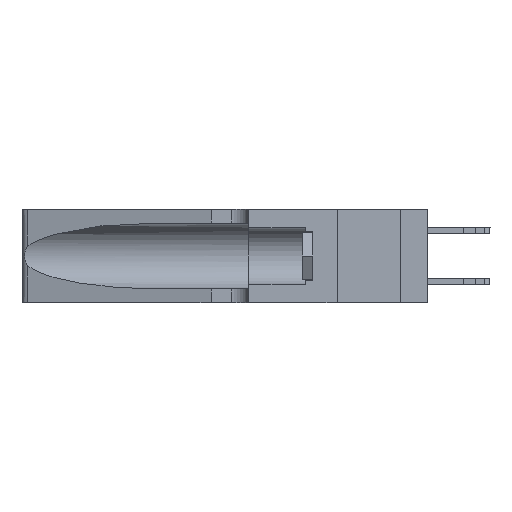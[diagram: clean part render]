
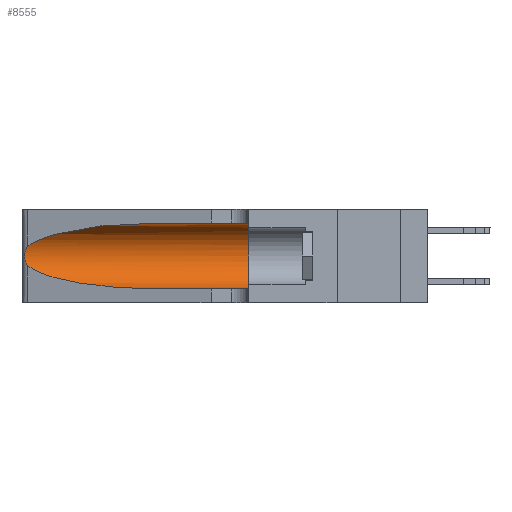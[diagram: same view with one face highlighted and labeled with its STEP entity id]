
A CAD part, left-side view. The second image highlights one B-rep face of the part: STEP entity #8555.
In plain terms, the highlighted cylindrical face has radius 3.308 mm (diameter 6.617 mm), a partial arc.
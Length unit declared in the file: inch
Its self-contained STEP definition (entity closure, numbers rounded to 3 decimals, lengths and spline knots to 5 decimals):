
#260 = CARTESIAN_POINT ( 'NONE',  ( 0.25639, 1.23186, 0.15144 ) ) ;
#756 = AXIS2_PLACEMENT_3D ( 'NONE', #12316, #9847, #24020 ) ;
#944 = VECTOR ( 'NONE', #30191, 39.37008 ) ;
#1982 = EDGE_CURVE ( 'NONE', #26042, #21639, #18127, .T. ) ;
#2422 = CARTESIAN_POINT ( 'NONE',  ( 0.25787, 1.23484, 0.2124 ) ) ;
#2727 = CARTESIAN_POINT ( 'NONE',  ( 0.25639, 1.23184, 0.21858 ) ) ;
#3432 = FACE_OUTER_BOUND ( 'NONE', #24597, .T. ) ;
#3894 = VERTEX_POINT ( 'NONE', #22502 ) ;
#4821 = CARTESIAN_POINT ( 'NONE',  ( 0.26075, 1.23896, 0.178 ) ) ;
#6118 = EDGE_CURVE ( 'NONE', #26042, #29046, #21059, .T. ) ;
#6675 = CARTESIAN_POINT ( 'NONE',  ( 0.2373, 1.15595, 0.28018 ) ) ;
#7386 = CARTESIAN_POINT ( 'NONE',  ( 0.25555, 1.22994, 0.2215 ) ) ;
#7749 = DIRECTION ( 'NONE',  ( 0., 0., -1. ) ) ;
#8228 = CARTESIAN_POINT ( 'NONE',  ( 0.1305, 0.72297, 0.31525 ) ) ;
#8555 = ADVANCED_FACE ( 'NONE', ( #3432 ), #15640, .F. ) ;
#9847 = DIRECTION ( 'NONE',  ( 0., 1., 0. ) ) ;
#10007 = VECTOR ( 'NONE', #13375, 39.37008 ) ;
#10968 = ORIENTED_EDGE ( 'NONE', *, *, #30305, .F. ) ;
#11940 = CARTESIAN_POINT ( 'NONE',  ( 0.26018, 1.23835, 0.19895 ) ) ;
#12041 = CARTESIAN_POINT ( 'NONE',  ( 0.26017, 1.23833, 0.17102 ) ) ;
#12077 = CARTESIAN_POINT ( 'NONE',  ( 0.25487, 1.22718, 0.22369 ) ) ;
#12197 = CARTESIAN_POINT ( 'NONE',  ( 0.2373, 1.15595, 0.08982 ) ) ;
#12316 = CARTESIAN_POINT ( 'NONE',  ( 0.1305, 0.35, 0.185 ) ) ;
#12512 = ORIENTED_EDGE ( 'NONE', *, *, #27457, .T. ) ;
#13101 = EDGE_CURVE ( 'NONE', #3894, #23990, #29773, .T. ) ;
#13375 = DIRECTION ( 'NONE',  ( 0., -1., 0. ) ) ;
#14307 = CARTESIAN_POINT ( 'NONE',  ( 0.25856, 1.23593, 0.16098 ) ) ;
#14887 = CARTESIAN_POINT ( 'NONE',  ( 0.1305, 1.61858, 0.185 ) ) ;
#14941 = ORIENTED_EDGE ( 'NONE', *, *, #13101, .T. ) ;
#15640 = CYLINDRICAL_SURFACE ( 'NONE', #25316, 0.13025 ) ;
#16698 = CARTESIAN_POINT ( 'NONE',  ( 0.25789, 1.23486, 0.15765 ) ) ;
#17646 = VERTEX_POINT ( 'NONE', #18879 ) ;
#18127 = LINE ( 'NONE', #25194, #10007 ) ;
#18879 = CARTESIAN_POINT ( 'NONE',  ( 0.1305, 0.35, 0.05475 ) ) ;
#19049 = B_SPLINE_CURVE_WITH_KNOTS ( 'NONE', 3,
 ( #28723, #7386, #2727, #2422, #19100, #11940, #19301, #4821, #12041, #14307, #16698, #260, #21687, #23845 ),
 .UNSPECIFIED., .F., .F.,
 ( 4, 2, 2, 2, 2, 2, 4 ),
 ( 0., 0.00027, 0.00053, 0.00107, 0.0016, 0.00187, 0.00214 ),
 .UNSPECIFIED. ) ;
#19100 = CARTESIAN_POINT ( 'NONE',  ( 0.25854, 1.2359, 0.20912 ) ) ;
#19301 = CARTESIAN_POINT ( 'NONE',  ( 0.26075, 1.23896, 0.19203 ) ) ;
#19317 = ORIENTED_EDGE ( 'NONE', *, *, #25510, .T. ) ;
#19349 = CARTESIAN_POINT ( 'NONE',  ( 0.18966, 0.96281, 0.05475 ) ) ;
#20085 = ORIENTED_EDGE ( 'NONE', *, *, #6118, .T. ) ;
#20572 = CARTESIAN_POINT ( 'NONE',  ( 0.1305, 1.61858, 0.05475 ) ) ;
#21059 =( BOUNDED_CURVE ( )  B_SPLINE_CURVE ( 3, ( #21366, #29432, #6675, #12077 ),
 .UNSPECIFIED., .F., .F. ) 
 B_SPLINE_CURVE_WITH_KNOTS ( ( 4, 4 ),
 ( 1.5708, 2.84003 ),
 .UNSPECIFIED. ) 
 CURVE ( )  GEOMETRIC_REPRESENTATION_ITEM ( )  RATIONAL_B_SPLINE_CURVE ( ( 1., 0.87, 0.87, 1. ) ) 
 REPRESENTATION_ITEM ( '' )  );
#21066 = CARTESIAN_POINT ( 'NONE',  ( 0.1305, 0.35, 0.31525 ) ) ;
#21366 = CARTESIAN_POINT ( 'NONE',  ( 0.1305, 0.72297, 0.31525 ) ) ;
#21639 = VERTEX_POINT ( 'NONE', #21066 ) ;
#21687 = CARTESIAN_POINT ( 'NONE',  ( 0.25555, 1.22993, 0.14849 ) ) ;
#22040 = DIRECTION ( 'NONE',  ( 0., -1., 0. ) ) ;
#22502 = CARTESIAN_POINT ( 'NONE',  ( 0.25487, 1.22718, 0.14631 ) ) ;
#22517 = CARTESIAN_POINT ( 'NONE',  ( 0.1305, 0.72297, 0.05475 ) ) ;
#23600 = ORIENTED_EDGE ( 'NONE', *, *, #1982, .F. ) ;
#23845 = CARTESIAN_POINT ( 'NONE',  ( 0.25487, 1.22718, 0.14631 ) ) ;
#23990 = VERTEX_POINT ( 'NONE', #22517 ) ;
#24020 = DIRECTION ( 'NONE',  ( 0., 0., 1. ) ) ;
#24597 = EDGE_LOOP ( 'NONE', ( #20085, #12512, #14941, #19317, #10968, #23600 ) ) ;
#25128 = CARTESIAN_POINT ( 'NONE',  ( 0.25487, 1.22718, 0.22369 ) ) ;
#25194 = CARTESIAN_POINT ( 'NONE',  ( 0.1305, 1.61858, 0.31525 ) ) ;
#25316 = AXIS2_PLACEMENT_3D ( 'NONE', #14887, #22040, #7749 ) ;
#25510 = EDGE_CURVE ( 'NONE', #23990, #17646, #26127, .T. ) ;
#26042 = VERTEX_POINT ( 'NONE', #8228 ) ;
#26127 = LINE ( 'NONE', #20572, #944 ) ;
#26282 = CARTESIAN_POINT ( 'NONE',  ( 0.25487, 1.22718, 0.14631 ) ) ;
#27015 = CARTESIAN_POINT ( 'NONE',  ( 0.1305, 0.72297, 0.05475 ) ) ;
#27457 = EDGE_CURVE ( 'NONE', #29046, #3894, #19049, .T. ) ;
#27875 = CIRCLE ( 'NONE', #756, 0.13025 ) ;
#28723 = CARTESIAN_POINT ( 'NONE',  ( 0.25487, 1.22718, 0.22369 ) ) ;
#29046 = VERTEX_POINT ( 'NONE', #25128 ) ;
#29432 = CARTESIAN_POINT ( 'NONE',  ( 0.18966, 0.96281, 0.31525 ) ) ;
#29773 =( BOUNDED_CURVE ( )  B_SPLINE_CURVE ( 3, ( #26282, #12197, #19349, #27015 ),
 .UNSPECIFIED., .F., .T. ) 
 B_SPLINE_CURVE_WITH_KNOTS ( ( 4, 4 ),
 ( 3.44316, 4.71239 ),
 .UNSPECIFIED. ) 
 CURVE ( )  GEOMETRIC_REPRESENTATION_ITEM ( )  RATIONAL_B_SPLINE_CURVE ( ( 1., 0.87, 0.87, 1. ) ) 
 REPRESENTATION_ITEM ( '' )  );
#30191 = DIRECTION ( 'NONE',  ( 0., -1., 0. ) ) ;
#30305 = EDGE_CURVE ( 'NONE', #21639, #17646, #27875, .T. ) ;
